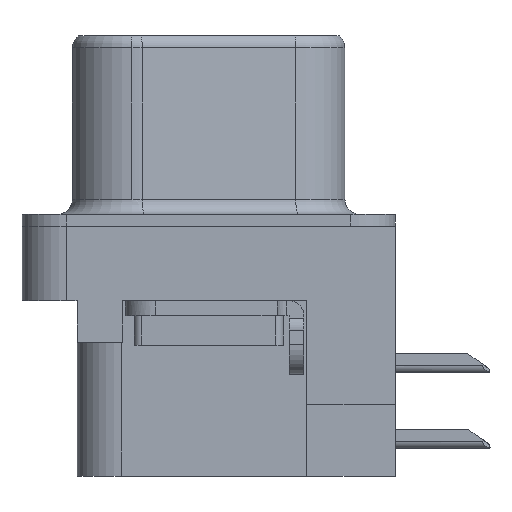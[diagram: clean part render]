
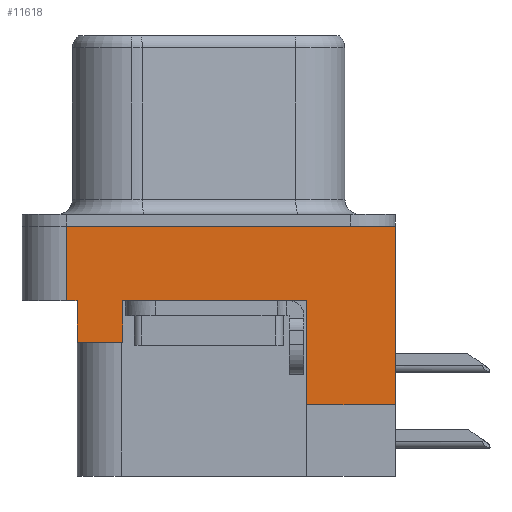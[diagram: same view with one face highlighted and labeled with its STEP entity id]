
A CAD part, left-side view. The second image highlights one B-rep face of the part: STEP entity #11618.
In plain terms, the highlighted planar face has unit normal (-1, 0, 0).
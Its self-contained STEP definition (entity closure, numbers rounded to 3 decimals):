
#35 = VERTEX_POINT ( 'NONE', #8914 ) ;
#284 = CARTESIAN_POINT ( 'NONE',  ( -2.935, 4.775, -2.5 ) ) ;
#706 = VECTOR ( 'NONE', #7683, 1000. ) ;
#930 = DIRECTION ( 'NONE',  ( 0., 0., 1. ) ) ;
#971 = CARTESIAN_POINT ( 'NONE',  ( -2.935, 2.895, -2.5 ) ) ;
#991 = ORIENTED_EDGE ( 'NONE', *, *, #3875, .F. ) ;
#1227 = FACE_OUTER_BOUND ( 'NONE', #7746, .T. ) ;
#1506 = CARTESIAN_POINT ( 'NONE',  ( -2.935, 4.425, -2.5 ) ) ;
#2212 = CARTESIAN_POINT ( 'NONE',  ( -2.935, -3.295, -8.4 ) ) ;
#2537 = VECTOR ( 'NONE', #11602, 1000. ) ;
#2544 = ORIENTED_EDGE ( 'NONE', *, *, #10438, .T. ) ;
#2564 = LINE ( 'NONE', #15969, #2537 ) ;
#2631 = LINE ( 'NONE', #284, #15995 ) ;
#2705 = CARTESIAN_POINT ( 'NONE',  ( -2.935, 2.895, -3.9 ) ) ;
#3182 = VECTOR ( 'NONE', #14542, 1000. ) ;
#3293 = EDGE_CURVE ( 'NONE', #12106, #11700, #4333, .T. ) ;
#3556 = VERTEX_POINT ( 'NONE', #4429 ) ;
#3762 = EDGE_CURVE ( 'NONE', #15365, #8805, #7908, .T. ) ;
#3791 = EDGE_CURVE ( 'NONE', #8338, #3556, #2631, .T. ) ;
#3875 = EDGE_CURVE ( 'NONE', #3556, #7272, #5431, .T. ) ;
#3894 = EDGE_CURVE ( 'NONE', #12106, #7272, #12820, .T. ) ;
#4333 = LINE ( 'NONE', #13930, #3182 ) ;
#4429 = CARTESIAN_POINT ( 'NONE',  ( -2.935, 4.775, 0. ) ) ;
#4509 = CARTESIAN_POINT ( 'NONE',  ( -2.935, -6.275, -2.5 ) ) ;
#4598 = DIRECTION ( 'NONE',  ( 0., 0., 1. ) ) ;
#4707 = EDGE_CURVE ( 'NONE', #11700, #5180, #4896, .T. ) ;
#4896 = LINE ( 'NONE', #2212, #8250 ) ;
#4982 = VECTOR ( 'NONE', #17527, 1000. ) ;
#5010 = VECTOR ( 'NONE', #11391, 1000. ) ;
#5060 = LINE ( 'NONE', #2705, #5010 ) ;
#5076 = DIRECTION ( 'NONE',  ( 0., -1., 0. ) ) ;
#5180 = VERTEX_POINT ( 'NONE', #5213 ) ;
#5197 = VECTOR ( 'NONE', #17785, 1000. ) ;
#5213 = CARTESIAN_POINT ( 'NONE',  ( -2.935, -3.295, -2.5 ) ) ;
#5301 = CARTESIAN_POINT ( 'NONE',  ( -2.935, -6.275, -6. ) ) ;
#5431 = LINE ( 'NONE', #14954, #5197 ) ;
#5633 = CARTESIAN_POINT ( 'NONE',  ( -2.935, -6.275, -2.5 ) ) ;
#5803 = ORIENTED_EDGE ( 'NONE', *, *, #3293, .F. ) ;
#6040 = EDGE_CURVE ( 'NONE', #8338, #8805, #12783, .T. ) ;
#6691 = ORIENTED_EDGE ( 'NONE', *, *, #17902, .F. ) ;
#6794 = VECTOR ( 'NONE', #14178, 1000. ) ;
#6982 = PLANE ( 'NONE',  #17950 ) ;
#7043 = CARTESIAN_POINT ( 'NONE',  ( -2.935, 4.425, -3.9 ) ) ;
#7050 = DIRECTION ( 'NONE',  ( -1., 0., 0. ) ) ;
#7144 = CARTESIAN_POINT ( 'NONE',  ( -2.935, 4.775, -2.5 ) ) ;
#7174 = LINE ( 'NONE', #8330, #6794 ) ;
#7272 = VERTEX_POINT ( 'NONE', #13121 ) ;
#7433 = ORIENTED_EDGE ( 'NONE', *, *, #3762, .F. ) ;
#7683 = DIRECTION ( 'NONE',  ( 0., 0., 1. ) ) ;
#7746 = EDGE_LOOP ( 'NONE', ( #5803, #14497, #991, #10387, #17020, #7433, #6691, #2544, #14305, #18172 ) ) ;
#7908 = LINE ( 'NONE', #7043, #706 ) ;
#8250 = VECTOR ( 'NONE', #930, 1000. ) ;
#8330 = CARTESIAN_POINT ( 'NONE',  ( -2.935, -6.275, -2.5 ) ) ;
#8338 = VERTEX_POINT ( 'NONE', #7144 ) ;
#8805 = VERTEX_POINT ( 'NONE', #1506 ) ;
#8914 = CARTESIAN_POINT ( 'NONE',  ( -2.935, 2.895, -3.9 ) ) ;
#9589 = CARTESIAN_POINT ( 'NONE',  ( -2.935, 4.425, -3.9 ) ) ;
#10048 = EDGE_CURVE ( 'NONE', #11996, #5180, #7174, .T. ) ;
#10387 = ORIENTED_EDGE ( 'NONE', *, *, #3791, .F. ) ;
#10438 = EDGE_CURVE ( 'NONE', #35, #11996, #5060, .T. ) ;
#11391 = DIRECTION ( 'NONE',  ( 0., 0., 1. ) ) ;
#11602 = DIRECTION ( 'NONE',  ( 0., 1., 0. ) ) ;
#11618 = ADVANCED_FACE ( 'NONE', ( #1227 ), #6982, .T. ) ;
#11700 = VERTEX_POINT ( 'NONE', #14552 ) ;
#11996 = VERTEX_POINT ( 'NONE', #971 ) ;
#12106 = VERTEX_POINT ( 'NONE', #5301 ) ;
#12783 = LINE ( 'NONE', #4509, #13903 ) ;
#12820 = LINE ( 'NONE', #17415, #4982 ) ;
#13121 = CARTESIAN_POINT ( 'NONE',  ( -2.935, -6.275, 0. ) ) ;
#13903 = VECTOR ( 'NONE', #5076, 1000. ) ;
#13930 = CARTESIAN_POINT ( 'NONE',  ( -2.935, -6.495, -6. ) ) ;
#14178 = DIRECTION ( 'NONE',  ( 0., -1., 0. ) ) ;
#14305 = ORIENTED_EDGE ( 'NONE', *, *, #10048, .T. ) ;
#14497 = ORIENTED_EDGE ( 'NONE', *, *, #3894, .T. ) ;
#14542 = DIRECTION ( 'NONE',  ( 0., 1., 0. ) ) ;
#14552 = CARTESIAN_POINT ( 'NONE',  ( -2.935, -3.295, -6. ) ) ;
#14954 = CARTESIAN_POINT ( 'NONE',  ( -2.935, -6.275, 0. ) ) ;
#15365 = VERTEX_POINT ( 'NONE', #9589 ) ;
#15969 = CARTESIAN_POINT ( 'NONE',  ( -2.935, 4.425, -3.9 ) ) ;
#15995 = VECTOR ( 'NONE', #4598, 1000. ) ;
#17020 = ORIENTED_EDGE ( 'NONE', *, *, #6040, .T. ) ;
#17204 = DIRECTION ( 'NONE',  ( 0., 0., 1. ) ) ;
#17415 = CARTESIAN_POINT ( 'NONE',  ( -2.935, -6.275, -2.5 ) ) ;
#17527 = DIRECTION ( 'NONE',  ( 0., 0., 1. ) ) ;
#17785 = DIRECTION ( 'NONE',  ( 0., -1., 0. ) ) ;
#17902 = EDGE_CURVE ( 'NONE', #35, #15365, #2564, .T. ) ;
#17950 = AXIS2_PLACEMENT_3D ( 'NONE', #5633, #7050, #17204 ) ;
#18172 = ORIENTED_EDGE ( 'NONE', *, *, #4707, .F. ) ;
